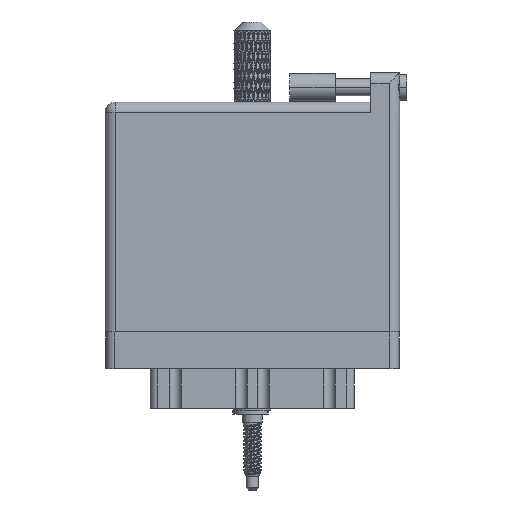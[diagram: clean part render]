
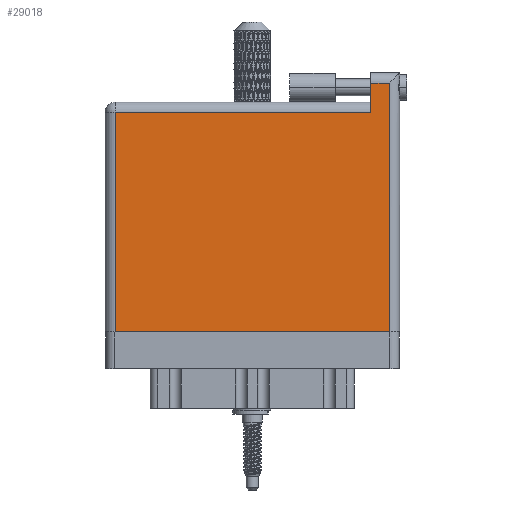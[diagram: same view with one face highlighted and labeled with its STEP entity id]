
A CAD part, front view. The second image highlights one B-rep face of the part: STEP entity #29018.
In plain terms, the highlighted face is planar.
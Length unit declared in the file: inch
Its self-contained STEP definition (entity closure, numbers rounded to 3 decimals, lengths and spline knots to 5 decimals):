
#758 = VECTOR ( 'NONE', #45431, 39.37008 ) ;
#3447 = CARTESIAN_POINT ( 'NONE',  ( 1.938, 1.696, 0. ) ) ;
#3981 = EDGE_CURVE ( 'NONE', #49824, #9541, #95980, .T. ) ;
#7810 = ORIENTED_EDGE ( 'NONE', *, *, #80867, .T. ) ;
#8753 = CARTESIAN_POINT ( 'NONE',  ( 0., 1.566, 0. ) ) ;
#9541 = VERTEX_POINT ( 'NONE', #45204 ) ;
#10862 = ORIENTED_EDGE ( 'NONE', *, *, #56353, .T. ) ;
#20133 = VECTOR ( 'NONE', #38236, 39.37008 ) ;
#21338 = ORIENTED_EDGE ( 'NONE', *, *, #61428, .T. ) ;
#21503 = CARTESIAN_POINT ( 'NONE',  ( 0., 1.496, 0. ) ) ;
#22378 = LINE ( 'NONE', #95784, #20133 ) ;
#24771 = CARTESIAN_POINT ( 'NONE',  ( 0.07, 0., 0. ) ) ;
#26682 = PLANE ( 'NONE',  #85773 ) ;
#27744 = VECTOR ( 'NONE', #36813, 39.37008 ) ;
#29018 = ADVANCED_FACE ( 'NONE', ( #48919 ), #26682, .F. ) ;
#31851 = VERTEX_POINT ( 'NONE', #73724 ) ;
#34110 = DIRECTION ( 'NONE',  ( 0., 0., -1. ) ) ;
#34613 = ORIENTED_EDGE ( 'NONE', *, *, #58265, .T. ) ;
#35705 = LINE ( 'NONE', #51020, #70713 ) ;
#36813 = DIRECTION ( 'NONE',  ( 0., -1., 0. ) ) ;
#37529 = LINE ( 'NONE', #70750, #758 ) ;
#38236 = DIRECTION ( 'NONE',  ( 0., -1., 0. ) ) ;
#42814 = ORIENTED_EDGE ( 'NONE', *, *, #3981, .T. ) ;
#45204 = CARTESIAN_POINT ( 'NONE',  ( 0.07, 1.496, 0. ) ) ;
#45431 = DIRECTION ( 'NONE',  ( -1., 0., 0. ) ) ;
#48919 = FACE_OUTER_BOUND ( 'NONE', #55617, .T. ) ;
#49824 = VERTEX_POINT ( 'NONE', #51760 ) ;
#51020 = CARTESIAN_POINT ( 'NONE',  ( 0., 0., 0. ) ) ;
#51519 = CARTESIAN_POINT ( 'NONE',  ( 1.938, 1.766, 0. ) ) ;
#51760 = CARTESIAN_POINT ( 'NONE',  ( 1.811, 1.496, 0. ) ) ;
#52655 = LINE ( 'NONE', #69009, #27744 ) ;
#54258 = DIRECTION ( 'NONE',  ( -1., 0., 0. ) ) ;
#55617 = EDGE_LOOP ( 'NONE', ( #10862, #21338, #7810, #77267, #42814, #34613 ) ) ;
#56353 = EDGE_CURVE ( 'NONE', #61768, #31851, #35705, .T. ) ;
#58265 = EDGE_CURVE ( 'NONE', #9541, #61768, #22378, .T. ) ;
#58954 = DIRECTION ( 'NONE',  ( 1., 0., 0. ) ) ;
#60861 = VECTOR ( 'NONE', #101108, 39.37008 ) ;
#61428 = EDGE_CURVE ( 'NONE', #31851, #78200, #84723, .T. ) ;
#61768 = VERTEX_POINT ( 'NONE', #24771 ) ;
#66442 = VECTOR ( 'NONE', #54258, 39.37008 ) ;
#67760 = CARTESIAN_POINT ( 'NONE',  ( 1.811, 1.696, 0. ) ) ;
#69009 = CARTESIAN_POINT ( 'NONE',  ( 1.811, 1.766, 0. ) ) ;
#70713 = VECTOR ( 'NONE', #58954, 39.37008 ) ;
#70750 = CARTESIAN_POINT ( 'NONE',  ( 0., 1.696, 0. ) ) ;
#73724 = CARTESIAN_POINT ( 'NONE',  ( 1.938, 0., 0. ) ) ;
#74057 = VERTEX_POINT ( 'NONE', #67760 ) ;
#77267 = ORIENTED_EDGE ( 'NONE', *, *, #81463, .T. ) ;
#78200 = VERTEX_POINT ( 'NONE', #3447 ) ;
#80867 = EDGE_CURVE ( 'NONE', #78200, #74057, #37529, .T. ) ;
#81463 = EDGE_CURVE ( 'NONE', #74057, #49824, #52655, .T. ) ;
#83167 = DIRECTION ( 'NONE',  ( -1., 0., 0. ) ) ;
#84723 = LINE ( 'NONE', #51519, #60861 ) ;
#85773 = AXIS2_PLACEMENT_3D ( 'NONE', #8753, #34110, #83167 ) ;
#95784 = CARTESIAN_POINT ( 'NONE',  ( 0.07, 0., 0. ) ) ;
#95980 = LINE ( 'NONE', #21503, #66442 ) ;
#101108 = DIRECTION ( 'NONE',  ( 0., 1., 0. ) ) ;
